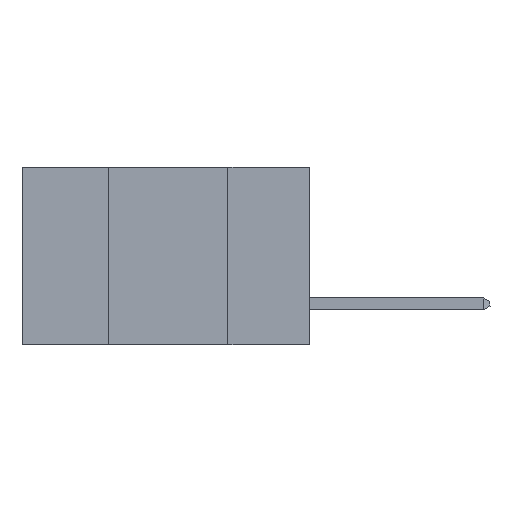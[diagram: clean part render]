
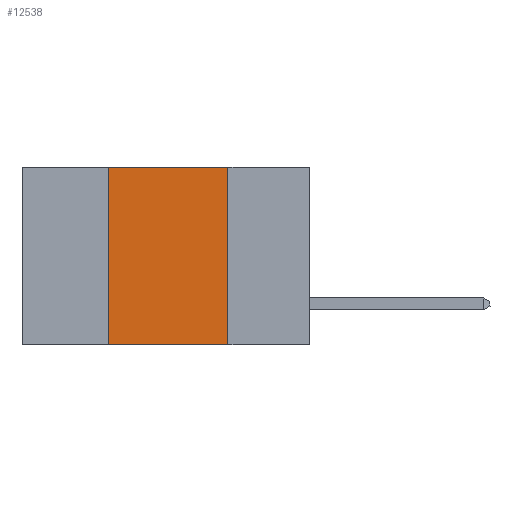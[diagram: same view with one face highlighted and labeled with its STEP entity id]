
A CAD part, left-side view. The second image highlights one B-rep face of the part: STEP entity #12538.
In plain terms, the highlighted planar face has unit normal (-1, 0, 0).
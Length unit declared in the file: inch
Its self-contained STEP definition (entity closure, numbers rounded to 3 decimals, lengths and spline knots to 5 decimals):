
#389 = ORIENTED_EDGE ( 'NONE', *, *, #8801, .F. ) ;
#1235 = DIRECTION ( 'NONE',  ( 1., 0., 0. ) ) ;
#1359 = VERTEX_POINT ( 'NONE', #12997 ) ;
#1526 = DIRECTION ( 'NONE',  ( 0., 0., 1. ) ) ;
#2208 = EDGE_CURVE ( 'NONE', #8191, #1359, #9296, .T. ) ;
#2214 = VERTEX_POINT ( 'NONE', #8238 ) ;
#2380 = CARTESIAN_POINT ( 'NONE',  ( 0., 0.6, -0.37 ) ) ;
#4559 = DIRECTION ( 'NONE',  ( 0., -1., 0. ) ) ;
#5109 = EDGE_LOOP ( 'NONE', ( #16819, #15709, #389, #16478 ) ) ;
#5226 = PLANE ( 'NONE',  #8751 ) ;
#5472 = VECTOR ( 'NONE', #1526, 39.37008 ) ;
#7530 = LINE ( 'NONE', #14408, #5472 ) ;
#8074 = LINE ( 'NONE', #2380, #12581 ) ;
#8089 = VECTOR ( 'NONE', #9207, 39.37008 ) ;
#8149 = CARTESIAN_POINT ( 'NONE',  ( 0., 0.42, 0. ) ) ;
#8191 = VERTEX_POINT ( 'NONE', #8149 ) ;
#8238 = CARTESIAN_POINT ( 'NONE',  ( 0., 0.17, -0.37 ) ) ;
#8751 = AXIS2_PLACEMENT_3D ( 'NONE', #13073, #1235, #10583 ) ;
#8801 = EDGE_CURVE ( 'NONE', #11100, #8191, #7530, .T. ) ;
#9207 = DIRECTION ( 'NONE',  ( 0., 0., -1. ) ) ;
#9296 = LINE ( 'NONE', #10904, #9905 ) ;
#9905 = VECTOR ( 'NONE', #4559, 39.37008 ) ;
#10268 = CARTESIAN_POINT ( 'NONE',  ( 0., 0.42, -0.37 ) ) ;
#10583 = DIRECTION ( 'NONE',  ( 0., 0., -1. ) ) ;
#10904 = CARTESIAN_POINT ( 'NONE',  ( 0., 0.6, 0. ) ) ;
#11100 = VERTEX_POINT ( 'NONE', #10268 ) ;
#11523 = DIRECTION ( 'NONE',  ( 0., -1., 0. ) ) ;
#12538 = ADVANCED_FACE ( 'NONE', ( #14144 ), #5226, .F. ) ;
#12581 = VECTOR ( 'NONE', #11523, 39.37008 ) ;
#12997 = CARTESIAN_POINT ( 'NONE',  ( 0., 0.17, 0. ) ) ;
#13073 = CARTESIAN_POINT ( 'NONE',  ( 0., 0.6, 0. ) ) ;
#13413 = LINE ( 'NONE', #15495, #8089 ) ;
#14144 = FACE_OUTER_BOUND ( 'NONE', #5109, .T. ) ;
#14408 = CARTESIAN_POINT ( 'NONE',  ( 0., 0.42, 0. ) ) ;
#15495 = CARTESIAN_POINT ( 'NONE',  ( 0., 0.17, 0. ) ) ;
#15676 = EDGE_CURVE ( 'NONE', #1359, #2214, #13413, .T. ) ;
#15709 = ORIENTED_EDGE ( 'NONE', *, *, #2208, .F. ) ;
#16112 = EDGE_CURVE ( 'NONE', #11100, #2214, #8074, .T. ) ;
#16478 = ORIENTED_EDGE ( 'NONE', *, *, #16112, .T. ) ;
#16819 = ORIENTED_EDGE ( 'NONE', *, *, #15676, .F. ) ;
